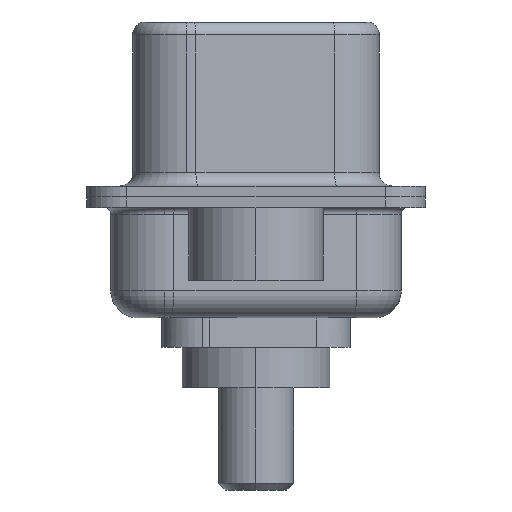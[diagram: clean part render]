
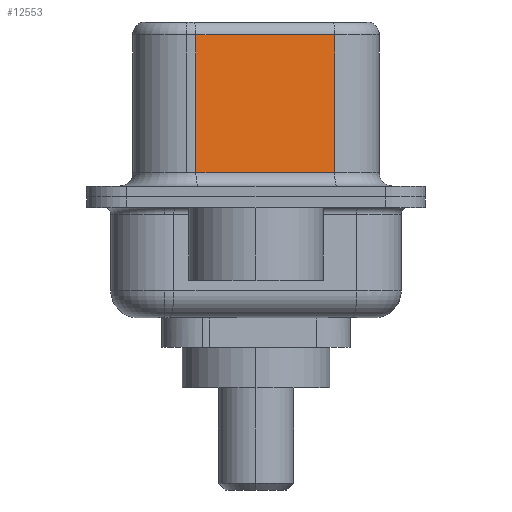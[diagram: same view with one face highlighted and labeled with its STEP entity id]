
A CAD part, left-side view. The second image highlights one B-rep face of the part: STEP entity #12553.
In plain terms, the highlighted planar face has unit normal (-0.985, -0.174, 0).
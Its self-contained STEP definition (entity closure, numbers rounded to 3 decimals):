
#288 = EDGE_CURVE ( 'NONE', #2930, #7618, #1786, .T. ) ;
#519 = DIRECTION ( 'NONE',  ( 0., 0., -1. ) ) ;
#663 = VERTEX_POINT ( 'NONE', #1242 ) ;
#732 = CARTESIAN_POINT ( 'NONE',  ( 4.565, -2.927, 6.02 ) ) ;
#789 = DIRECTION ( 'NONE',  ( 0., 0., -1. ) ) ;
#899 = LINE ( 'NONE', #732, #10242 ) ;
#1242 = CARTESIAN_POINT ( 'NONE',  ( 4.565, -2.927, 6.02 ) ) ;
#1723 = ORIENTED_EDGE ( 'NONE', *, *, #15018, .T. ) ;
#1786 = LINE ( 'NONE', #5029, #4679 ) ;
#2617 = ORIENTED_EDGE ( 'NONE', *, *, #11172, .T. ) ;
#2930 = VERTEX_POINT ( 'NONE', #7863 ) ;
#3915 = ORIENTED_EDGE ( 'NONE', *, *, #11216, .F. ) ;
#3921 = DIRECTION ( 'NONE',  ( 0.985, 0.174, 0. ) ) ;
#4048 = AXIS2_PLACEMENT_3D ( 'NONE', #11001, #3921, #12232 ) ;
#4679 = VECTOR ( 'NONE', #519, 1000. ) ;
#5029 = CARTESIAN_POINT ( 'NONE',  ( 3.655, 2.233, 6.52 ) ) ;
#5869 = ORIENTED_EDGE ( 'NONE', *, *, #288, .T. ) ;
#6623 = VERTEX_POINT ( 'NONE', #12666 ) ;
#6950 = CARTESIAN_POINT ( 'NONE',  ( 4.565, -2.927, 0.9 ) ) ;
#7083 = VECTOR ( 'NONE', #789, 1000. ) ;
#7506 = CARTESIAN_POINT ( 'NONE',  ( 3.655, 2.233, 0.9 ) ) ;
#7618 = VERTEX_POINT ( 'NONE', #7506 ) ;
#7863 = CARTESIAN_POINT ( 'NONE',  ( 3.655, 2.233, 6.02 ) ) ;
#8191 = LINE ( 'NONE', #13984, #7083 ) ;
#8337 = FACE_OUTER_BOUND ( 'NONE', #9334, .T. ) ;
#9321 = DIRECTION ( 'NONE',  ( -0.174, 0.985, 0. ) ) ;
#9334 = EDGE_LOOP ( 'NONE', ( #3915, #1723, #5869, #2617 ) ) ;
#10242 = VECTOR ( 'NONE', #9321, 1000. ) ;
#11001 = CARTESIAN_POINT ( 'NONE',  ( 4.565, -2.927, 6.52 ) ) ;
#11172 = EDGE_CURVE ( 'NONE', #7618, #6623, #14321, .T. ) ;
#11216 = EDGE_CURVE ( 'NONE', #663, #6623, #8191, .T. ) ;
#12232 = DIRECTION ( 'NONE',  ( -0.174, 0.985, 0. ) ) ;
#12553 = ADVANCED_FACE ( 'NONE', ( #8337 ), #13348, .F. ) ;
#12666 = CARTESIAN_POINT ( 'NONE',  ( 4.565, -2.927, 0.9 ) ) ;
#12720 = DIRECTION ( 'NONE',  ( 0.174, -0.985, 0. ) ) ;
#13348 = PLANE ( 'NONE',  #4048 ) ;
#13984 = CARTESIAN_POINT ( 'NONE',  ( 4.565, -2.927, 6.52 ) ) ;
#14321 = LINE ( 'NONE', #6950, #15058 ) ;
#15018 = EDGE_CURVE ( 'NONE', #663, #2930, #899, .T. ) ;
#15058 = VECTOR ( 'NONE', #12720, 1000. ) ;
